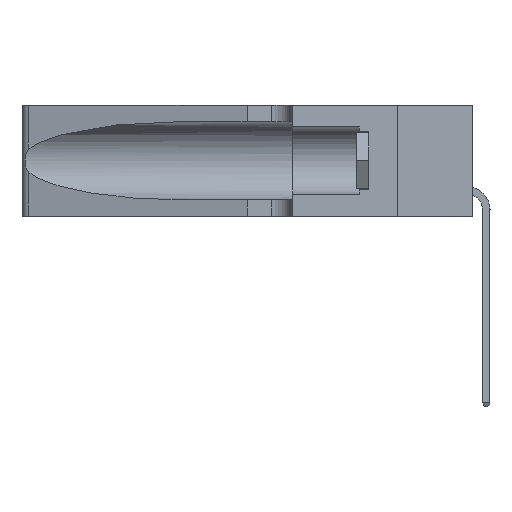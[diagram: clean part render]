
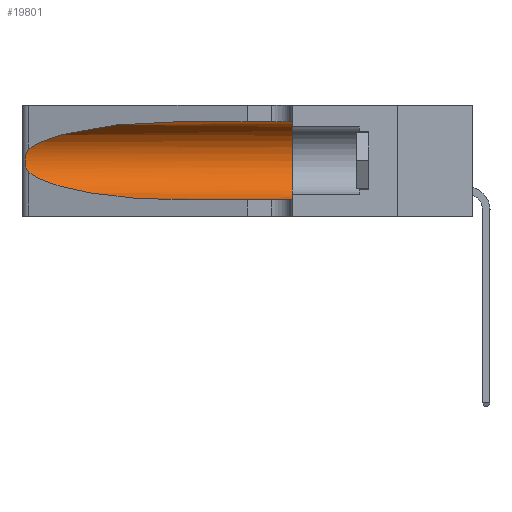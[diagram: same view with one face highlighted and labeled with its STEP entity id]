
A CAD part, left-side view. The second image highlights one B-rep face of the part: STEP entity #19801.
In plain terms, the highlighted cylindrical face has radius 3.308 mm (diameter 6.617 mm), a partial arc.
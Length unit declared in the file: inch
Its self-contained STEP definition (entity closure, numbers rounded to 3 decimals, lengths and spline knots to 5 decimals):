
#828 = CARTESIAN_POINT ( 'NONE',  ( 0.18966, 0.96281, 0.31525 ) ) ;
#1824 = CARTESIAN_POINT ( 'NONE',  ( 0.25487, 1.22718, 0.14631 ) ) ;
#3519 = EDGE_CURVE ( 'NONE', #11745, #27007, #38477, .T. ) ;
#5270 = CARTESIAN_POINT ( 'NONE',  ( 0.26018, 1.23835, 0.19895 ) ) ;
#5848 = CARTESIAN_POINT ( 'NONE',  ( 0.25789, 1.23486, 0.15765 ) ) ;
#6185 = ORIENTED_EDGE ( 'NONE', *, *, #44649, .F. ) ;
#6661 = VERTEX_POINT ( 'NONE', #7465 ) ;
#6947 = CARTESIAN_POINT ( 'NONE',  ( 0.26017, 1.23833, 0.17102 ) ) ;
#6981 = DIRECTION ( 'NONE',  ( 0., 1., 0. ) ) ;
#7413 = CARTESIAN_POINT ( 'NONE',  ( 0.26075, 1.23896, 0.178 ) ) ;
#7456 = LINE ( 'NONE', #43546, #11917 ) ;
#7465 = CARTESIAN_POINT ( 'NONE',  ( 0.25487, 1.22718, 0.14631 ) ) ;
#11745 = VERTEX_POINT ( 'NONE', #12149 ) ;
#11917 = VECTOR ( 'NONE', #40137, 39.37008 ) ;
#12149 = CARTESIAN_POINT ( 'NONE',  ( 0.1305, 0.72297, 0.05475 ) ) ;
#12203 = VERTEX_POINT ( 'NONE', #14508 ) ;
#12754 = CARTESIAN_POINT ( 'NONE',  ( 0.25555, 1.22994, 0.2215 ) ) ;
#13139 = DIRECTION ( 'NONE',  ( 0., -1., 0. ) ) ;
#13328 = ORIENTED_EDGE ( 'NONE', *, *, #26556, .F. ) ;
#13456 = EDGE_LOOP ( 'NONE', ( #29445, #31630, #37245, #15773, #13328, #6185 ) ) ;
#14508 = CARTESIAN_POINT ( 'NONE',  ( 0.25487, 1.22718, 0.22369 ) ) ;
#14842 = CARTESIAN_POINT ( 'NONE',  ( 0.25487, 1.22718, 0.14631 ) ) ;
#15217 = CARTESIAN_POINT ( 'NONE',  ( 0.25487, 1.22718, 0.22369 ) ) ;
#15773 = ORIENTED_EDGE ( 'NONE', *, *, #3519, .T. ) ;
#16065 = CARTESIAN_POINT ( 'NONE',  ( 0.25856, 1.23593, 0.16098 ) ) ;
#16572 = B_SPLINE_CURVE_WITH_KNOTS ( 'NONE', 3,
 ( #33532, #12754, #21587, #40411, #28044, #5270, #36098, #7413, #6947, #16065, #5848, #30692, #40686, #1824 ),
 .UNSPECIFIED., .F., .F.,
 ( 4, 2, 2, 2, 2, 2, 4 ),
 ( 0., 0.00027, 0.00053, 0.00107, 0.0016, 0.00187, 0.00214 ),
 .UNSPECIFIED. ) ;
#16966 = CARTESIAN_POINT ( 'NONE',  ( 0.1305, 0.35, 0.05475 ) ) ;
#17042 = CYLINDRICAL_SURFACE ( 'NONE', #40308, 0.13025 ) ;
#18480 = DIRECTION ( 'NONE',  ( 0., -1., 0. ) ) ;
#19465 = VERTEX_POINT ( 'NONE', #44115 ) ;
#19801 = ADVANCED_FACE ( 'NONE', ( #26445 ), #17042, .F. ) ;
#21256 = AXIS2_PLACEMENT_3D ( 'NONE', #28115, #6981, #28258 ) ;
#21587 = CARTESIAN_POINT ( 'NONE',  ( 0.25639, 1.23184, 0.21858 ) ) ;
#21973 = CARTESIAN_POINT ( 'NONE',  ( 0.1305, 0.72297, 0.31525 ) ) ;
#22246 = CARTESIAN_POINT ( 'NONE',  ( 0.1305, 0.72297, 0.05475 ) ) ;
#23240 = CIRCLE ( 'NONE', #21256, 0.13025 ) ;
#25417 = EDGE_CURVE ( 'NONE', #6661, #11745, #37178, .T. ) ;
#26445 = FACE_OUTER_BOUND ( 'NONE', #13456, .T. ) ;
#26556 = EDGE_CURVE ( 'NONE', #19465, #27007, #23240, .T. ) ;
#27007 = VERTEX_POINT ( 'NONE', #16966 ) ;
#28044 = CARTESIAN_POINT ( 'NONE',  ( 0.25854, 1.2359, 0.20912 ) ) ;
#28115 = CARTESIAN_POINT ( 'NONE',  ( 0.1305, 0.35, 0.185 ) ) ;
#28258 = DIRECTION ( 'NONE',  ( 0., 0., 1. ) ) ;
#29445 = ORIENTED_EDGE ( 'NONE', *, *, #41643, .T. ) ;
#30692 = CARTESIAN_POINT ( 'NONE',  ( 0.25639, 1.23186, 0.15144 ) ) ;
#30728 = DIRECTION ( 'NONE',  ( 0., 0., -1. ) ) ;
#31630 = ORIENTED_EDGE ( 'NONE', *, *, #35782, .T. ) ;
#33532 = CARTESIAN_POINT ( 'NONE',  ( 0.25487, 1.22718, 0.22369 ) ) ;
#35782 = EDGE_CURVE ( 'NONE', #12203, #6661, #16572, .T. ) ;
#36098 = CARTESIAN_POINT ( 'NONE',  ( 0.26075, 1.23896, 0.19203 ) ) ;
#36250 = CARTESIAN_POINT ( 'NONE',  ( 0.2373, 1.15595, 0.08982 ) ) ;
#36338 = CARTESIAN_POINT ( 'NONE',  ( 0.1305, 1.61858, 0.05475 ) ) ;
#37178 =( BOUNDED_CURVE ( )  B_SPLINE_CURVE ( 3, ( #14842, #36250, #40112, #22246 ),
 .UNSPECIFIED., .F., .F. ) 
 B_SPLINE_CURVE_WITH_KNOTS ( ( 4, 4 ),
 ( 3.44316, 4.71239 ),
 .UNSPECIFIED. ) 
 CURVE ( )  GEOMETRIC_REPRESENTATION_ITEM ( )  RATIONAL_B_SPLINE_CURVE ( ( 1., 0.87, 0.87, 1. ) ) 
 REPRESENTATION_ITEM ( '' )  );
#37245 = ORIENTED_EDGE ( 'NONE', *, *, #25417, .T. ) ;
#37390 = VECTOR ( 'NONE', #18480, 39.37008 ) ;
#38477 = LINE ( 'NONE', #36338, #37390 ) ;
#38547 =( BOUNDED_CURVE ( )  B_SPLINE_CURVE ( 3, ( #21973, #828, #43242, #15217 ),
 .UNSPECIFIED., .F., .T. ) 
 B_SPLINE_CURVE_WITH_KNOTS ( ( 4, 4 ),
 ( 1.5708, 2.84003 ),
 .UNSPECIFIED. ) 
 CURVE ( )  GEOMETRIC_REPRESENTATION_ITEM ( )  RATIONAL_B_SPLINE_CURVE ( ( 1., 0.87, 0.87, 1. ) ) 
 REPRESENTATION_ITEM ( '' )  );
#40112 = CARTESIAN_POINT ( 'NONE',  ( 0.18966, 0.96281, 0.05475 ) ) ;
#40137 = DIRECTION ( 'NONE',  ( 0., -1., 0. ) ) ;
#40308 = AXIS2_PLACEMENT_3D ( 'NONE', #41321, #13139, #30728 ) ;
#40411 = CARTESIAN_POINT ( 'NONE',  ( 0.25787, 1.23484, 0.2124 ) ) ;
#40686 = CARTESIAN_POINT ( 'NONE',  ( 0.25555, 1.22993, 0.14849 ) ) ;
#41321 = CARTESIAN_POINT ( 'NONE',  ( 0.1305, 1.61858, 0.185 ) ) ;
#41643 = EDGE_CURVE ( 'NONE', #42340, #12203, #38547, .T. ) ;
#42340 = VERTEX_POINT ( 'NONE', #42555 ) ;
#42555 = CARTESIAN_POINT ( 'NONE',  ( 0.1305, 0.72297, 0.31525 ) ) ;
#43242 = CARTESIAN_POINT ( 'NONE',  ( 0.2373, 1.15595, 0.28018 ) ) ;
#43546 = CARTESIAN_POINT ( 'NONE',  ( 0.1305, 1.61858, 0.31525 ) ) ;
#44115 = CARTESIAN_POINT ( 'NONE',  ( 0.1305, 0.35, 0.31525 ) ) ;
#44649 = EDGE_CURVE ( 'NONE', #42340, #19465, #7456, .T. ) ;
